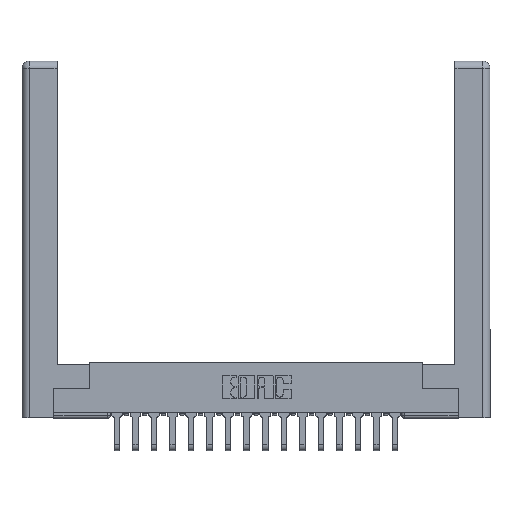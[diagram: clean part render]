
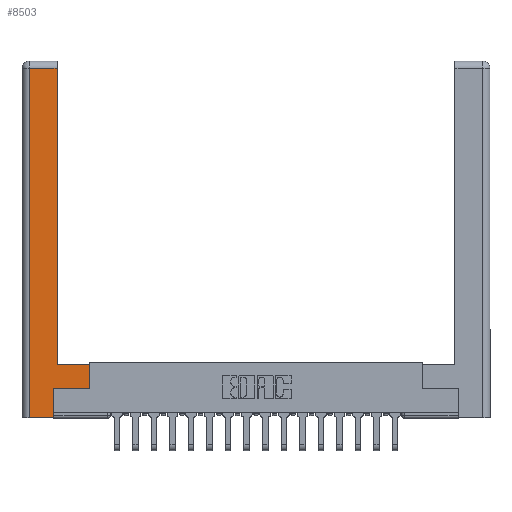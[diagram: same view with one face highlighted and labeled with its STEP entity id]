
A CAD part, top view. The second image highlights one B-rep face of the part: STEP entity #8503.
In plain terms, the highlighted planar face has unit normal (0, 0, 1).
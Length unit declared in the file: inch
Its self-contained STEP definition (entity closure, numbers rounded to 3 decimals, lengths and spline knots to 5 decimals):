
#1675 = DIRECTION ( 'NONE',  ( 0., -1., 0. ) ) ;
#2345 = CARTESIAN_POINT ( 'NONE',  ( 0.295, 0.45, 0. ) ) ;
#2468 = CARTESIAN_POINT ( 'NONE',  ( 0.295, 0.45, 0. ) ) ;
#2756 = CARTESIAN_POINT ( 'NONE',  ( 0.295, 3., 0. ) ) ;
#2838 = FACE_OUTER_BOUND ( 'NONE', #15809, .T. ) ;
#3577 = CARTESIAN_POINT ( 'NONE',  ( 0.565, 0.45, 0. ) ) ;
#3653 = DIRECTION ( 'NONE',  ( 0., 1., 0. ) ) ;
#3676 = EDGE_CURVE ( 'NONE', #10122, #12750, #15146, .T. ) ;
#3802 = DIRECTION ( 'NONE',  ( -1., 0., 0. ) ) ;
#4185 = ORIENTED_EDGE ( 'NONE', *, *, #3676, .T. ) ;
#4273 = CARTESIAN_POINT ( 'NONE',  ( 0.565, 0.45, 0. ) ) ;
#4604 = DIRECTION ( 'NONE',  ( 1., 0., 0. ) ) ;
#5236 = VERTEX_POINT ( 'NONE', #4273 ) ;
#5239 = CARTESIAN_POINT ( 'NONE',  ( 0.265, 0., 0. ) ) ;
#5650 = VERTEX_POINT ( 'NONE', #17372 ) ;
#5809 = ORIENTED_EDGE ( 'NONE', *, *, #15596, .T. ) ;
#5944 = ORIENTED_EDGE ( 'NONE', *, *, #12172, .T. ) ;
#6120 = VERTEX_POINT ( 'NONE', #15200 ) ;
#6477 = VERTEX_POINT ( 'NONE', #11220 ) ;
#6663 = EDGE_CURVE ( 'NONE', #5650, #6120, #15362, .T. ) ;
#6784 = CARTESIAN_POINT ( 'NONE',  ( 0.265, 0.245, 0. ) ) ;
#6826 = CARTESIAN_POINT ( 'NONE',  ( 0.0615, 0., 0. ) ) ;
#6999 = PLANE ( 'NONE',  #10607 ) ;
#7167 = VECTOR ( 'NONE', #4604, 39.37008 ) ;
#7494 = VECTOR ( 'NONE', #1675, 39.37008 ) ;
#8006 = LINE ( 'NONE', #6826, #7494 ) ;
#8503 = ADVANCED_FACE ( 'NONE', ( #2838 ), #6999, .F. ) ;
#8629 = CARTESIAN_POINT ( 'NONE',  ( 0.0615, 2.94, 0. ) ) ;
#9129 = ORIENTED_EDGE ( 'NONE', *, *, #6663, .T. ) ;
#10122 = VERTEX_POINT ( 'NONE', #5239 ) ;
#10251 = ORIENTED_EDGE ( 'NONE', *, *, #19170, .T. ) ;
#10265 = DIRECTION ( 'NONE',  ( 0., 0., -1. ) ) ;
#10607 = AXIS2_PLACEMENT_3D ( 'NONE', #12151, #10265, #13743 ) ;
#11220 = CARTESIAN_POINT ( 'NONE',  ( 0.0615, 0., 0. ) ) ;
#11783 = VECTOR ( 'NONE', #18101, 39.37008 ) ;
#11927 = LINE ( 'NONE', #2345, #12976 ) ;
#12151 = CARTESIAN_POINT ( 'NONE',  ( 0., 0., 0. ) ) ;
#12172 = EDGE_CURVE ( 'NONE', #19417, #5650, #16385, .T. ) ;
#12750 = VERTEX_POINT ( 'NONE', #14841 ) ;
#12811 = VECTOR ( 'NONE', #3653, 39.37008 ) ;
#12976 = VECTOR ( 'NONE', #20745, 39.37008 ) ;
#13044 = EDGE_CURVE ( 'NONE', #5236, #19417, #11927, .T. ) ;
#13142 = LINE ( 'NONE', #21217, #7167 ) ;
#13494 = EDGE_CURVE ( 'NONE', #6120, #6477, #8006, .T. ) ;
#13743 = DIRECTION ( 'NONE',  ( -1., 0., 0. ) ) ;
#14005 = VERTEX_POINT ( 'NONE', #19885 ) ;
#14841 = CARTESIAN_POINT ( 'NONE',  ( 0.265, 0.245, 0. ) ) ;
#15146 = LINE ( 'NONE', #6784, #11783 ) ;
#15200 = CARTESIAN_POINT ( 'NONE',  ( 0.0615, 2.94, 0. ) ) ;
#15362 = LINE ( 'NONE', #8629, #19543 ) ;
#15437 = ORIENTED_EDGE ( 'NONE', *, *, #19255, .T. ) ;
#15596 = EDGE_CURVE ( 'NONE', #12750, #14005, #13142, .T. ) ;
#15809 = EDGE_LOOP ( 'NONE', ( #5944, #9129, #20026, #10251, #4185, #5809, #15437, #20035 ) ) ;
#15951 = DIRECTION ( 'NONE',  ( 0., 1., 0. ) ) ;
#16385 = LINE ( 'NONE', #2756, #17712 ) ;
#17372 = CARTESIAN_POINT ( 'NONE',  ( 0.295, 2.94, 0. ) ) ;
#17712 = VECTOR ( 'NONE', #15951, 39.37008 ) ;
#18101 = DIRECTION ( 'NONE',  ( 0., 1., 0. ) ) ;
#18161 = CARTESIAN_POINT ( 'NONE',  ( 0.265, 0., 0. ) ) ;
#18802 = LINE ( 'NONE', #18161, #19557 ) ;
#19170 = EDGE_CURVE ( 'NONE', #6477, #10122, #18802, .T. ) ;
#19255 = EDGE_CURVE ( 'NONE', #14005, #5236, #19314, .T. ) ;
#19314 = LINE ( 'NONE', #3577, #12811 ) ;
#19417 = VERTEX_POINT ( 'NONE', #2468 ) ;
#19543 = VECTOR ( 'NONE', #3802, 39.37008 ) ;
#19545 = DIRECTION ( 'NONE',  ( 1., 0., 0. ) ) ;
#19557 = VECTOR ( 'NONE', #19545, 39.37008 ) ;
#19885 = CARTESIAN_POINT ( 'NONE',  ( 0.565, 0.245, 0. ) ) ;
#20026 = ORIENTED_EDGE ( 'NONE', *, *, #13494, .T. ) ;
#20035 = ORIENTED_EDGE ( 'NONE', *, *, #13044, .T. ) ;
#20745 = DIRECTION ( 'NONE',  ( -1., 0., 0. ) ) ;
#21217 = CARTESIAN_POINT ( 'NONE',  ( 0.565, 0.245, 0. ) ) ;
